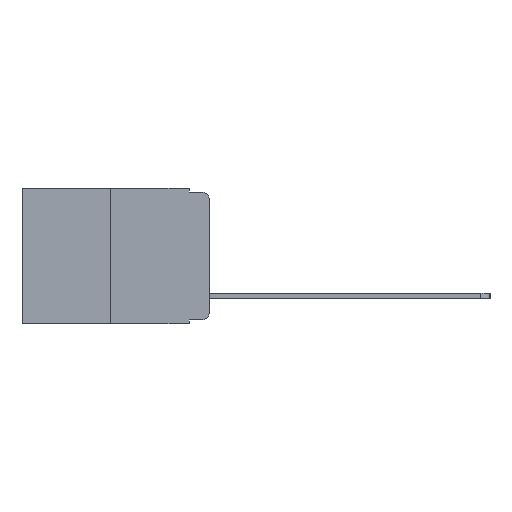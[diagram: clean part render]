
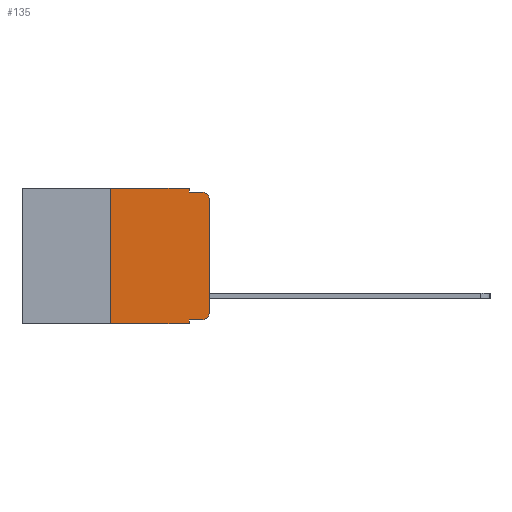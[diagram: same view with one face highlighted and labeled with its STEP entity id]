
A CAD part, left-side view. The second image highlights one B-rep face of the part: STEP entity #135.
In plain terms, the highlighted planar face has unit normal (-1, 0, 0).
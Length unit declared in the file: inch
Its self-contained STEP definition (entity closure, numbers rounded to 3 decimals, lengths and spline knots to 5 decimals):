
#64 = VERTEX_POINT ( 'NONE', #7331 ) ;
#135 = ADVANCED_FACE ( 'NONE', ( #1981 ), #7545, .F. ) ;
#310 = AXIS2_PLACEMENT_3D ( 'NONE', #9006, #8940, #10488 ) ;
#318 = CARTESIAN_POINT ( 'NONE',  ( 0., 0.473, -0.343 ) ) ;
#1234 = VECTOR ( 'NONE', #9851, 39.37008 ) ;
#1436 = ORIENTED_EDGE ( 'NONE', *, *, #7444, .F. ) ;
#1443 = CARTESIAN_POINT ( 'NONE',  ( 0., 0.051, -0.01 ) ) ;
#1607 = CIRCLE ( 'NONE', #11057, 0.02 ) ;
#1644 = VERTEX_POINT ( 'NONE', #5607 ) ;
#1819 = AXIS2_PLACEMENT_3D ( 'NONE', #12109, #5474, #13195 ) ;
#1955 = CARTESIAN_POINT ( 'NONE',  ( 0., 0., -0.313 ) ) ;
#1981 = FACE_OUTER_BOUND ( 'NONE', #8944, .T. ) ;
#2048 = CARTESIAN_POINT ( 'NONE',  ( 0., 0.473, 0. ) ) ;
#2141 = CARTESIAN_POINT ( 'NONE',  ( 0., 0.051, -0.343 ) ) ;
#2161 = CARTESIAN_POINT ( 'NONE',  ( 0., 0.051, 0. ) ) ;
#2185 = VECTOR ( 'NONE', #9659, 39.37008 ) ;
#2999 = LINE ( 'NONE', #1443, #2185 ) ;
#3020 = ORIENTED_EDGE ( 'NONE', *, *, #9715, .T. ) ;
#3365 = VECTOR ( 'NONE', #3905, 39.37008 ) ;
#3524 = LINE ( 'NONE', #9706, #6253 ) ;
#3837 = ORIENTED_EDGE ( 'NONE', *, *, #6708, .F. ) ;
#3905 = DIRECTION ( 'NONE',  ( 0., -1., 0. ) ) ;
#3929 = LINE ( 'NONE', #12132, #12474 ) ;
#4285 = VERTEX_POINT ( 'NONE', #6264 ) ;
#4361 = DIRECTION ( 'NONE',  ( 0., 0., 1. ) ) ;
#4411 = VERTEX_POINT ( 'NONE', #12008 ) ;
#4436 = EDGE_CURVE ( 'NONE', #64, #5571, #1607, .T. ) ;
#4566 = LINE ( 'NONE', #318, #1234 ) ;
#4732 = ORIENTED_EDGE ( 'NONE', *, *, #13082, .T. ) ;
#4745 = VECTOR ( 'NONE', #11254, 39.37008 ) ;
#4850 = CARTESIAN_POINT ( 'NONE',  ( 0., 0.051, -0.333 ) ) ;
#5100 = LINE ( 'NONE', #2048, #4745 ) ;
#5289 = ORIENTED_EDGE ( 'NONE', *, *, #5971, .T. ) ;
#5474 = DIRECTION ( 'NONE',  ( -1., 0., 0. ) ) ;
#5571 = VERTEX_POINT ( 'NONE', #1955 ) ;
#5607 = CARTESIAN_POINT ( 'NONE',  ( 0., 0.02, -0.01 ) ) ;
#5782 = ORIENTED_EDGE ( 'NONE', *, *, #10436, .T. ) ;
#5971 = EDGE_CURVE ( 'NONE', #6510, #64, #6452, .T. ) ;
#6253 = VECTOR ( 'NONE', #14028, 39.37008 ) ;
#6264 = CARTESIAN_POINT ( 'NONE',  ( 0., 0.25, -0.343 ) ) ;
#6328 = VECTOR ( 'NONE', #14100, 39.37008 ) ;
#6366 = ORIENTED_EDGE ( 'NONE', *, *, #4436, .T. ) ;
#6452 = LINE ( 'NONE', #10672, #3365 ) ;
#6510 = VERTEX_POINT ( 'NONE', #4850 ) ;
#6552 = DIRECTION ( 'NONE',  ( -1., 0., 0. ) ) ;
#6708 = EDGE_CURVE ( 'NONE', #6510, #7009, #3524, .T. ) ;
#6729 = CARTESIAN_POINT ( 'NONE',  ( 0., 0.051, 0. ) ) ;
#7009 = VERTEX_POINT ( 'NONE', #2141 ) ;
#7331 = CARTESIAN_POINT ( 'NONE',  ( 0., 0.02, -0.333 ) ) ;
#7444 = EDGE_CURVE ( 'NONE', #4285, #4411, #12533, .T. ) ;
#7545 = PLANE ( 'NONE',  #310 ) ;
#7602 = CARTESIAN_POINT ( 'NONE',  ( 0., 0., -0.03 ) ) ;
#7793 = DIRECTION ( 'NONE',  ( 0., 0., -1. ) ) ;
#8210 = EDGE_CURVE ( 'NONE', #8662, #10854, #9115, .T. ) ;
#8662 = VERTEX_POINT ( 'NONE', #2161 ) ;
#8940 = DIRECTION ( 'NONE',  ( 1., 0., 0. ) ) ;
#8944 = EDGE_LOOP ( 'NONE', ( #5782, #3020, #14892, #13389, #10844, #1436, #4732, #3837, #5289, #6366 ) ) ;
#8977 = EDGE_CURVE ( 'NONE', #10854, #1644, #2999, .T. ) ;
#8992 = CARTESIAN_POINT ( 'NONE',  ( 0., 0.051, -0.01 ) ) ;
#9006 = CARTESIAN_POINT ( 'NONE',  ( 0., 0.473, 0. ) ) ;
#9115 = LINE ( 'NONE', #6729, #14538 ) ;
#9659 = DIRECTION ( 'NONE',  ( 0., -1., 0. ) ) ;
#9706 = CARTESIAN_POINT ( 'NONE',  ( 0., 0.051, 0. ) ) ;
#9715 = EDGE_CURVE ( 'NONE', #13072, #1644, #13684, .T. ) ;
#9778 = CARTESIAN_POINT ( 'NONE',  ( 0., 0.25, 0. ) ) ;
#9851 = DIRECTION ( 'NONE',  ( 0., -1., 0. ) ) ;
#10436 = EDGE_CURVE ( 'NONE', #5571, #13072, #3929, .T. ) ;
#10488 = DIRECTION ( 'NONE',  ( 0., 0., -1. ) ) ;
#10672 = CARTESIAN_POINT ( 'NONE',  ( 0., 0.051, -0.333 ) ) ;
#10844 = ORIENTED_EDGE ( 'NONE', *, *, #13274, .F. ) ;
#10854 = VERTEX_POINT ( 'NONE', #8992 ) ;
#11057 = AXIS2_PLACEMENT_3D ( 'NONE', #13137, #6552, #14227 ) ;
#11254 = DIRECTION ( 'NONE',  ( 0., -1., 0. ) ) ;
#12008 = CARTESIAN_POINT ( 'NONE',  ( 0., 0.25, 0. ) ) ;
#12109 = CARTESIAN_POINT ( 'NONE',  ( 0., 0.02, -0.03 ) ) ;
#12132 = CARTESIAN_POINT ( 'NONE',  ( 0., 0., 0. ) ) ;
#12474 = VECTOR ( 'NONE', #4361, 39.37008 ) ;
#12533 = LINE ( 'NONE', #9778, #6328 ) ;
#13072 = VERTEX_POINT ( 'NONE', #7602 ) ;
#13082 = EDGE_CURVE ( 'NONE', #4285, #7009, #4566, .T. ) ;
#13137 = CARTESIAN_POINT ( 'NONE',  ( 0., 0.02, -0.313 ) ) ;
#13195 = DIRECTION ( 'NONE',  ( 0., 0., -1. ) ) ;
#13274 = EDGE_CURVE ( 'NONE', #4411, #8662, #5100, .T. ) ;
#13389 = ORIENTED_EDGE ( 'NONE', *, *, #8210, .F. ) ;
#13684 = CIRCLE ( 'NONE', #1819, 0.02 ) ;
#14028 = DIRECTION ( 'NONE',  ( 0., 0., -1. ) ) ;
#14100 = DIRECTION ( 'NONE',  ( 0., 0., 1. ) ) ;
#14227 = DIRECTION ( 'NONE',  ( 0., 0., -1. ) ) ;
#14538 = VECTOR ( 'NONE', #7793, 39.37008 ) ;
#14892 = ORIENTED_EDGE ( 'NONE', *, *, #8977, .F. ) ;
